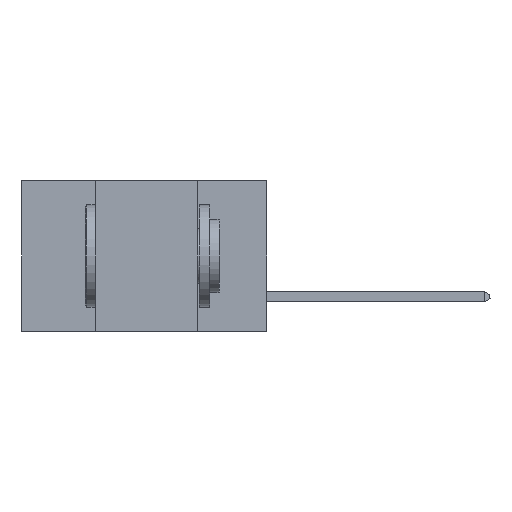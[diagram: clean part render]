
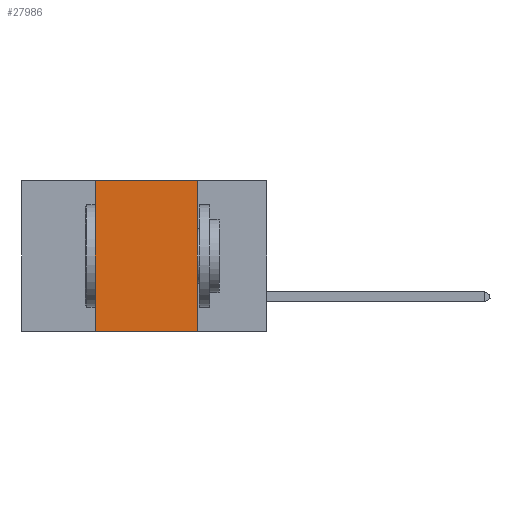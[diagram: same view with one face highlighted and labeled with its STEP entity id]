
A CAD part, left-side view. The second image highlights one B-rep face of the part: STEP entity #27986.
In plain terms, the highlighted planar face has unit normal (-1, 0, 0).
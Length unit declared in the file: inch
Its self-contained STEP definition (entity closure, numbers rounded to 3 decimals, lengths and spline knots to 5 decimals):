
#1384 = VECTOR ( 'NONE', #31851, 39.37008 ) ;
#1448 = VERTEX_POINT ( 'NONE', #41936 ) ;
#3092 = LINE ( 'NONE', #41151, #25124 ) ;
#4524 = FACE_OUTER_BOUND ( 'NONE', #36611, .T. ) ;
#4716 = ORIENTED_EDGE ( 'NONE', *, *, #31240, .T. ) ;
#6693 = LINE ( 'NONE', #29341, #21048 ) ;
#7779 = ORIENTED_EDGE ( 'NONE', *, *, #10631, .F. ) ;
#8767 = DIRECTION ( 'NONE',  ( 0., 0., -1. ) ) ;
#9010 = CARTESIAN_POINT ( 'NONE',  ( 0., 0.17, -0.37 ) ) ;
#9153 = CARTESIAN_POINT ( 'NONE',  ( 0., 0.17, 0. ) ) ;
#9240 = VERTEX_POINT ( 'NONE', #9010 ) ;
#9718 = DIRECTION ( 'NONE',  ( 0., 0., 1. ) ) ;
#10631 = EDGE_CURVE ( 'NONE', #28013, #40071, #39638, .T. ) ;
#11475 = DIRECTION ( 'NONE',  ( 1., 0., 0. ) ) ;
#15752 = ORIENTED_EDGE ( 'NONE', *, *, #20939, .F. ) ;
#19078 = CARTESIAN_POINT ( 'NONE',  ( 0., 0.6, 0. ) ) ;
#19549 = EDGE_CURVE ( 'NONE', #1448, #28013, #6693, .T. ) ;
#20939 = EDGE_CURVE ( 'NONE', #40071, #9240, #3092, .T. ) ;
#21048 = VECTOR ( 'NONE', #9718, 39.37008 ) ;
#21145 = LINE ( 'NONE', #30114, #29800 ) ;
#22123 = CARTESIAN_POINT ( 'NONE',  ( 0., 0.42, 0. ) ) ;
#25124 = VECTOR ( 'NONE', #41576, 39.37008 ) ;
#27830 = CARTESIAN_POINT ( 'NONE',  ( 0., 0.6, 0. ) ) ;
#27986 = ADVANCED_FACE ( 'NONE', ( #4524 ), #41052, .F. ) ;
#28013 = VERTEX_POINT ( 'NONE', #22123 ) ;
#29341 = CARTESIAN_POINT ( 'NONE',  ( 0., 0.42, 0. ) ) ;
#29800 = VECTOR ( 'NONE', #37315, 39.37008 ) ;
#30114 = CARTESIAN_POINT ( 'NONE',  ( 0., 0.6, -0.37 ) ) ;
#31240 = EDGE_CURVE ( 'NONE', #1448, #9240, #21145, .T. ) ;
#31851 = DIRECTION ( 'NONE',  ( 0., -1., 0. ) ) ;
#35645 = ORIENTED_EDGE ( 'NONE', *, *, #19549, .F. ) ;
#36611 = EDGE_LOOP ( 'NONE', ( #15752, #7779, #35645, #4716 ) ) ;
#37315 = DIRECTION ( 'NONE',  ( 0., -1., 0. ) ) ;
#39492 = AXIS2_PLACEMENT_3D ( 'NONE', #27830, #11475, #8767 ) ;
#39638 = LINE ( 'NONE', #19078, #1384 ) ;
#40071 = VERTEX_POINT ( 'NONE', #9153 ) ;
#41052 = PLANE ( 'NONE',  #39492 ) ;
#41151 = CARTESIAN_POINT ( 'NONE',  ( 0., 0.17, 0. ) ) ;
#41576 = DIRECTION ( 'NONE',  ( 0., 0., -1. ) ) ;
#41936 = CARTESIAN_POINT ( 'NONE',  ( 0., 0.42, -0.37 ) ) ;
